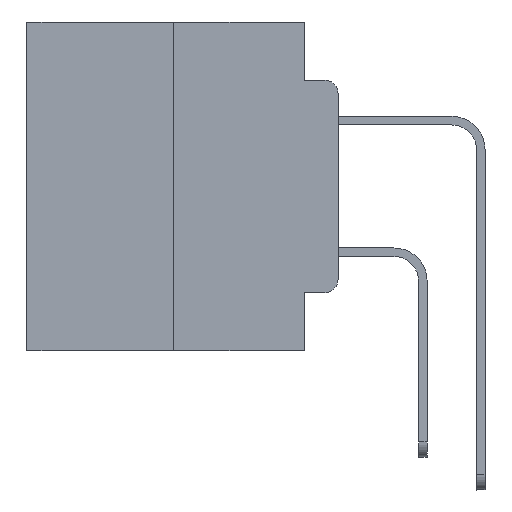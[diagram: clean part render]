
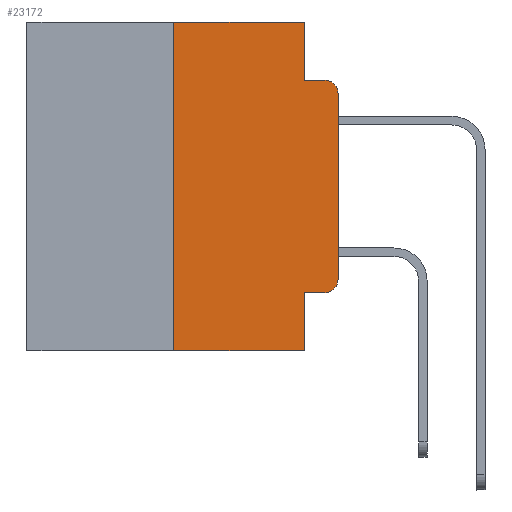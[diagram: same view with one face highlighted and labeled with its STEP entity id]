
A CAD part, left-side view. The second image highlights one B-rep face of the part: STEP entity #23172.
In plain terms, the highlighted planar face has unit normal (-1, 0, 0).
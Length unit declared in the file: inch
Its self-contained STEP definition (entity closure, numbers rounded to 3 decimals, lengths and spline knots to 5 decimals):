
#78 = VERTEX_POINT ( 'NONE', #26724 ) ;
#112 = ORIENTED_EDGE ( 'NONE', *, *, #20295, .F. ) ;
#343 = DIRECTION ( 'NONE',  ( 0., 0., -1. ) ) ;
#991 = ORIENTED_EDGE ( 'NONE', *, *, #21720, .T. ) ;
#1775 = VECTOR ( 'NONE', #343, 39.37008 ) ;
#1984 = ORIENTED_EDGE ( 'NONE', *, *, #24479, .T. ) ;
#2515 = VECTOR ( 'NONE', #19657, 39.37008 ) ;
#2776 = LINE ( 'NONE', #8903, #8050 ) ;
#3340 = DIRECTION ( 'NONE',  ( 1., 0., 0. ) ) ;
#3667 = VERTEX_POINT ( 'NONE', #20553 ) ;
#3810 = ORIENTED_EDGE ( 'NONE', *, *, #17486, .F. ) ;
#4673 = CARTESIAN_POINT ( 'NONE',  ( 0., 0.473, -0.5 ) ) ;
#4759 = CARTESIAN_POINT ( 'NONE',  ( 0., 0.051, -0.5 ) ) ;
#4866 = CARTESIAN_POINT ( 'NONE',  ( 0., 0.051, -0.0885 ) ) ;
#5773 = VECTOR ( 'NONE', #16847, 39.37008 ) ;
#5855 = CARTESIAN_POINT ( 'NONE',  ( 0., 0.051, -0.0885 ) ) ;
#6620 = VERTEX_POINT ( 'NONE', #5855 ) ;
#7792 = AXIS2_PLACEMENT_3D ( 'NONE', #12737, #27338, #14858 ) ;
#7850 = ORIENTED_EDGE ( 'NONE', *, *, #10802, .T. ) ;
#7885 = CARTESIAN_POINT ( 'NONE',  ( 0., 0., -0.1085 ) ) ;
#8050 = VECTOR ( 'NONE', #25792, 39.37008 ) ;
#8054 = CARTESIAN_POINT ( 'NONE',  ( 0., 0.051, 0. ) ) ;
#8220 = CARTESIAN_POINT ( 'NONE',  ( 0., 0.02, -0.0885 ) ) ;
#8343 = LINE ( 'NONE', #13576, #18276 ) ;
#8378 = ORIENTED_EDGE ( 'NONE', *, *, #14658, .F. ) ;
#8426 = LINE ( 'NONE', #13461, #1775 ) ;
#8466 = LINE ( 'NONE', #4673, #2515 ) ;
#8903 = CARTESIAN_POINT ( 'NONE',  ( 0., 0.051, -0.4115 ) ) ;
#9993 = ORIENTED_EDGE ( 'NONE', *, *, #11181, .F. ) ;
#10433 = EDGE_CURVE ( 'NONE', #17496, #21059, #19066, .T. ) ;
#10802 = EDGE_CURVE ( 'NONE', #3667, #10882, #8466, .T. ) ;
#10882 = VERTEX_POINT ( 'NONE', #4759 ) ;
#11181 = EDGE_CURVE ( 'NONE', #17978, #20440, #14091, .T. ) ;
#11304 = VECTOR ( 'NONE', #15595, 39.37008 ) ;
#11831 = EDGE_CURVE ( 'NONE', #78, #17496, #2776, .T. ) ;
#12032 = DIRECTION ( 'NONE',  ( -1., 0., 0. ) ) ;
#12737 = CARTESIAN_POINT ( 'NONE',  ( 0., 0.02, -0.1085 ) ) ;
#12836 = VERTEX_POINT ( 'NONE', #7885 ) ;
#13461 = CARTESIAN_POINT ( 'NONE',  ( 0., 0.051, 0. ) ) ;
#13576 = CARTESIAN_POINT ( 'NONE',  ( 0., 0.25, 0. ) ) ;
#14091 = LINE ( 'NONE', #23577, #24565 ) ;
#14191 = CARTESIAN_POINT ( 'NONE',  ( 0., 0.473, 0. ) ) ;
#14623 = FACE_OUTER_BOUND ( 'NONE', #16915, .T. ) ;
#14658 = EDGE_CURVE ( 'NONE', #78, #10882, #8426, .T. ) ;
#14708 = CARTESIAN_POINT ( 'NONE',  ( 0., 0., -0.3915 ) ) ;
#14768 = CARTESIAN_POINT ( 'NONE',  ( 0., 0., 0. ) ) ;
#14858 = DIRECTION ( 'NONE',  ( 0., 0., -1. ) ) ;
#15067 = VECTOR ( 'NONE', #26897, 39.37008 ) ;
#15074 = VERTEX_POINT ( 'NONE', #8220 ) ;
#15132 = CARTESIAN_POINT ( 'NONE',  ( 0., 0.25, 0. ) ) ;
#15595 = DIRECTION ( 'NONE',  ( 0., -1., 0. ) ) ;
#15664 = DIRECTION ( 'NONE',  ( 0., 0., 1. ) ) ;
#16045 = EDGE_CURVE ( 'NONE', #3667, #17978, #8343, .T. ) ;
#16509 = AXIS2_PLACEMENT_3D ( 'NONE', #14191, #3340, #18418 ) ;
#16847 = DIRECTION ( 'NONE',  ( 0., 0., 1. ) ) ;
#16915 = EDGE_LOOP ( 'NONE', ( #1984, #991, #3810, #112, #9993, #22855, #7850, #8378, #22560, #17281 ) ) ;
#17141 = LINE ( 'NONE', #14768, #5773 ) ;
#17281 = ORIENTED_EDGE ( 'NONE', *, *, #10433, .T. ) ;
#17486 = EDGE_CURVE ( 'NONE', #6620, #15074, #23118, .T. ) ;
#17496 = VERTEX_POINT ( 'NONE', #24055 ) ;
#17978 = VERTEX_POINT ( 'NONE', #15132 ) ;
#18276 = VECTOR ( 'NONE', #15664, 39.37008 ) ;
#18326 = PLANE ( 'NONE',  #16509 ) ;
#18418 = DIRECTION ( 'NONE',  ( 0., 0., -1. ) ) ;
#19066 = CIRCLE ( 'NONE', #23688, 0.02 ) ;
#19657 = DIRECTION ( 'NONE',  ( 0., -1., 0. ) ) ;
#20295 = EDGE_CURVE ( 'NONE', #20440, #6620, #26188, .T. ) ;
#20440 = VERTEX_POINT ( 'NONE', #27403 ) ;
#20553 = CARTESIAN_POINT ( 'NONE',  ( 0., 0.25, -0.5 ) ) ;
#21059 = VERTEX_POINT ( 'NONE', #14708 ) ;
#21720 = EDGE_CURVE ( 'NONE', #12836, #15074, #25166, .T. ) ;
#22560 = ORIENTED_EDGE ( 'NONE', *, *, #11831, .T. ) ;
#22855 = ORIENTED_EDGE ( 'NONE', *, *, #16045, .F. ) ;
#23118 = LINE ( 'NONE', #4866, #11304 ) ;
#23172 = ADVANCED_FACE ( 'NONE', ( #14623 ), #18326, .F. ) ;
#23577 = CARTESIAN_POINT ( 'NONE',  ( 0., 0.473, 0. ) ) ;
#23688 = AXIS2_PLACEMENT_3D ( 'NONE', #24586, #12032, #26652 ) ;
#24055 = CARTESIAN_POINT ( 'NONE',  ( 0., 0.02, -0.4115 ) ) ;
#24479 = EDGE_CURVE ( 'NONE', #21059, #12836, #17141, .T. ) ;
#24565 = VECTOR ( 'NONE', #25648, 39.37008 ) ;
#24586 = CARTESIAN_POINT ( 'NONE',  ( 0., 0.02, -0.3915 ) ) ;
#25166 = CIRCLE ( 'NONE', #7792, 0.02 ) ;
#25648 = DIRECTION ( 'NONE',  ( 0., -1., 0. ) ) ;
#25792 = DIRECTION ( 'NONE',  ( 0., -1., 0. ) ) ;
#26188 = LINE ( 'NONE', #8054, #15067 ) ;
#26652 = DIRECTION ( 'NONE',  ( 0., 0., -1. ) ) ;
#26724 = CARTESIAN_POINT ( 'NONE',  ( 0., 0.051, -0.4115 ) ) ;
#26897 = DIRECTION ( 'NONE',  ( 0., 0., -1. ) ) ;
#27338 = DIRECTION ( 'NONE',  ( -1., 0., 0. ) ) ;
#27403 = CARTESIAN_POINT ( 'NONE',  ( 0., 0.051, 0. ) ) ;
